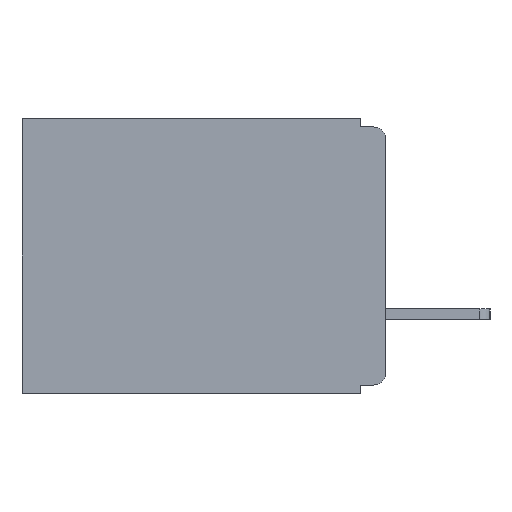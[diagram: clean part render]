
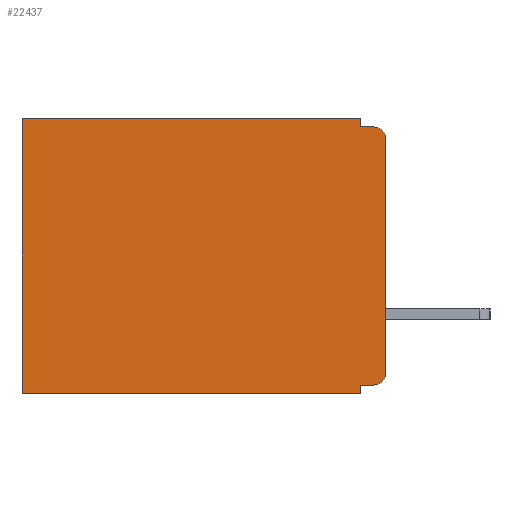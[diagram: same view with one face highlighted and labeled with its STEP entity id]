
A CAD part, left-side view. The second image highlights one B-rep face of the part: STEP entity #22437.
In plain terms, the highlighted planar face has unit normal (-1, 0, 0).
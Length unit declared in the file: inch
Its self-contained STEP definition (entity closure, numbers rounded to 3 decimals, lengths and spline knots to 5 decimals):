
#562 = VECTOR ( 'NONE', #17264, 39.37008 ) ;
#878 = DIRECTION ( 'NONE',  ( 0., 0., -1. ) ) ;
#922 = DIRECTION ( 'NONE',  ( 0., 1., 0. ) ) ;
#1477 = LINE ( 'NONE', #7710, #18221 ) ;
#1793 = AXIS2_PLACEMENT_3D ( 'NONE', #9737, #9732, #9717 ) ;
#2157 = DIRECTION ( 'NONE',  ( -1., 0., 0. ) ) ;
#2300 = VERTEX_POINT ( 'NONE', #17561 ) ;
#2523 = VECTOR ( 'NONE', #25443, 39.37008 ) ;
#3410 = ORIENTED_EDGE ( 'NONE', *, *, #23542, .T. ) ;
#3671 = VECTOR ( 'NONE', #922, 39.37008 ) ;
#3697 = ORIENTED_EDGE ( 'NONE', *, *, #10288, .T. ) ;
#3742 = ORIENTED_EDGE ( 'NONE', *, *, #21279, .F. ) ;
#4511 = ORIENTED_EDGE ( 'NONE', *, *, #25944, .F. ) ;
#6201 = EDGE_CURVE ( 'NONE', #26163, #18115, #25721, .T. ) ;
#6678 = CARTESIAN_POINT ( 'NONE',  ( 0.3, 0.015, -0.01 ) ) ;
#7618 = DIRECTION ( 'NONE',  ( 0., 0., -1. ) ) ;
#7710 = CARTESIAN_POINT ( 'NONE',  ( 0.3, 0.437, -0.33 ) ) ;
#8444 = CARTESIAN_POINT ( 'NONE',  ( 0.3, 0.031, 0. ) ) ;
#8586 = VERTEX_POINT ( 'NONE', #10783 ) ;
#8736 = PLANE ( 'NONE',  #22259 ) ;
#9625 = CARTESIAN_POINT ( 'NONE',  ( 0.3, 0.437, 0. ) ) ;
#9717 = DIRECTION ( 'NONE',  ( 0., 0., -1. ) ) ;
#9732 = DIRECTION ( 'NONE',  ( -1., 0., 0. ) ) ;
#9737 = CARTESIAN_POINT ( 'NONE',  ( 0.3, 0.015, -0.025 ) ) ;
#10111 = EDGE_CURVE ( 'NONE', #2300, #27895, #28093, .T. ) ;
#10136 = VERTEX_POINT ( 'NONE', #9625 ) ;
#10288 = EDGE_CURVE ( 'NONE', #10136, #18115, #1477, .T. ) ;
#10367 = ORIENTED_EDGE ( 'NONE', *, *, #13762, .F. ) ;
#10402 = CARTESIAN_POINT ( 'NONE',  ( 0.3, 0.031, -0.32 ) ) ;
#10783 = CARTESIAN_POINT ( 'NONE',  ( 0.3, 0., -0.305 ) ) ;
#10803 = LINE ( 'NONE', #13972, #22453 ) ;
#10963 = CARTESIAN_POINT ( 'NONE',  ( 0.3, 0., -0.33 ) ) ;
#11284 = AXIS2_PLACEMENT_3D ( 'NONE', #15199, #2157, #17401 ) ;
#13153 = DIRECTION ( 'NONE',  ( 0., 0., -1. ) ) ;
#13338 = EDGE_LOOP ( 'NONE', ( #4511, #16186, #10367, #18914, #23617, #3697, #20203, #3742, #20844, #3410 ) ) ;
#13762 = EDGE_CURVE ( 'NONE', #23883, #27895, #17998, .T. ) ;
#13972 = CARTESIAN_POINT ( 'NONE',  ( 0.3, 0.031, -0.33 ) ) ;
#14021 = CARTESIAN_POINT ( 'NONE',  ( 0.3, 0., 0. ) ) ;
#14075 = EDGE_CURVE ( 'NONE', #17575, #10136, #18035, .T. ) ;
#14305 = LINE ( 'NONE', #8444, #19419 ) ;
#14792 = VECTOR ( 'NONE', #19181, 39.37008 ) ;
#15199 = CARTESIAN_POINT ( 'NONE',  ( 0.3, 0.015, -0.305 ) ) ;
#15646 = CARTESIAN_POINT ( 'NONE',  ( 0.3, 0.015, -0.32 ) ) ;
#16186 = ORIENTED_EDGE ( 'NONE', *, *, #10111, .T. ) ;
#16818 = EDGE_CURVE ( 'NONE', #17801, #24912, #19931, .T. ) ;
#17264 = DIRECTION ( 'NONE',  ( 0., -1., 0. ) ) ;
#17401 = DIRECTION ( 'NONE',  ( 0., 0., -1. ) ) ;
#17561 = CARTESIAN_POINT ( 'NONE',  ( 0.3, 0., -0.025 ) ) ;
#17575 = VERTEX_POINT ( 'NONE', #27953 ) ;
#17714 = CARTESIAN_POINT ( 'NONE',  ( 0.3, 0., -0.33 ) ) ;
#17801 = VERTEX_POINT ( 'NONE', #15646 ) ;
#17998 = LINE ( 'NONE', #28125, #562 ) ;
#18035 = LINE ( 'NONE', #14021, #3671 ) ;
#18115 = VERTEX_POINT ( 'NONE', #25564 ) ;
#18221 = VECTOR ( 'NONE', #7618, 39.37008 ) ;
#18914 = ORIENTED_EDGE ( 'NONE', *, *, #20285, .F. ) ;
#19181 = DIRECTION ( 'NONE',  ( 0., 1., 0. ) ) ;
#19419 = VECTOR ( 'NONE', #21586, 39.37008 ) ;
#19931 = LINE ( 'NONE', #23277, #2523 ) ;
#20203 = ORIENTED_EDGE ( 'NONE', *, *, #6201, .F. ) ;
#20285 = EDGE_CURVE ( 'NONE', #17575, #23883, #14305, .T. ) ;
#20478 = CARTESIAN_POINT ( 'NONE',  ( 0.3, 0., -0.33 ) ) ;
#20741 = CARTESIAN_POINT ( 'NONE',  ( 0.3, 0.031, -0.01 ) ) ;
#20844 = ORIENTED_EDGE ( 'NONE', *, *, #16818, .F. ) ;
#21279 = EDGE_CURVE ( 'NONE', #24912, #26163, #10803, .T. ) ;
#21586 = DIRECTION ( 'NONE',  ( 0., 0., -1. ) ) ;
#22259 = AXIS2_PLACEMENT_3D ( 'NONE', #10963, #26226, #13153 ) ;
#22317 = FACE_OUTER_BOUND ( 'NONE', #13338, .T. ) ;
#22437 = ADVANCED_FACE ( 'NONE', ( #22317 ), #8736, .F. ) ;
#22453 = VECTOR ( 'NONE', #878, 39.37008 ) ;
#22707 = DIRECTION ( 'NONE',  ( 0., 0., -1. ) ) ;
#22804 = VECTOR ( 'NONE', #22707, 39.37008 ) ;
#23277 = CARTESIAN_POINT ( 'NONE',  ( 0.3, 0., -0.32 ) ) ;
#23478 = LINE ( 'NONE', #20478, #22804 ) ;
#23542 = EDGE_CURVE ( 'NONE', #17801, #8586, #27686, .T. ) ;
#23617 = ORIENTED_EDGE ( 'NONE', *, *, #14075, .T. ) ;
#23883 = VERTEX_POINT ( 'NONE', #20741 ) ;
#24912 = VERTEX_POINT ( 'NONE', #10402 ) ;
#25443 = DIRECTION ( 'NONE',  ( 0., 1., 0. ) ) ;
#25564 = CARTESIAN_POINT ( 'NONE',  ( 0.3, 0.437, -0.33 ) ) ;
#25721 = LINE ( 'NONE', #17714, #14792 ) ;
#25944 = EDGE_CURVE ( 'NONE', #2300, #8586, #23478, .T. ) ;
#26163 = VERTEX_POINT ( 'NONE', #27792 ) ;
#26226 = DIRECTION ( 'NONE',  ( 1., 0., 0. ) ) ;
#27686 = CIRCLE ( 'NONE', #11284, 0.015 ) ;
#27792 = CARTESIAN_POINT ( 'NONE',  ( 0.3, 0.031, -0.33 ) ) ;
#27895 = VERTEX_POINT ( 'NONE', #6678 ) ;
#27953 = CARTESIAN_POINT ( 'NONE',  ( 0.3, 0.031, 0. ) ) ;
#28093 = CIRCLE ( 'NONE', #1793, 0.015 ) ;
#28125 = CARTESIAN_POINT ( 'NONE',  ( 0.3, 0., -0.01 ) ) ;
